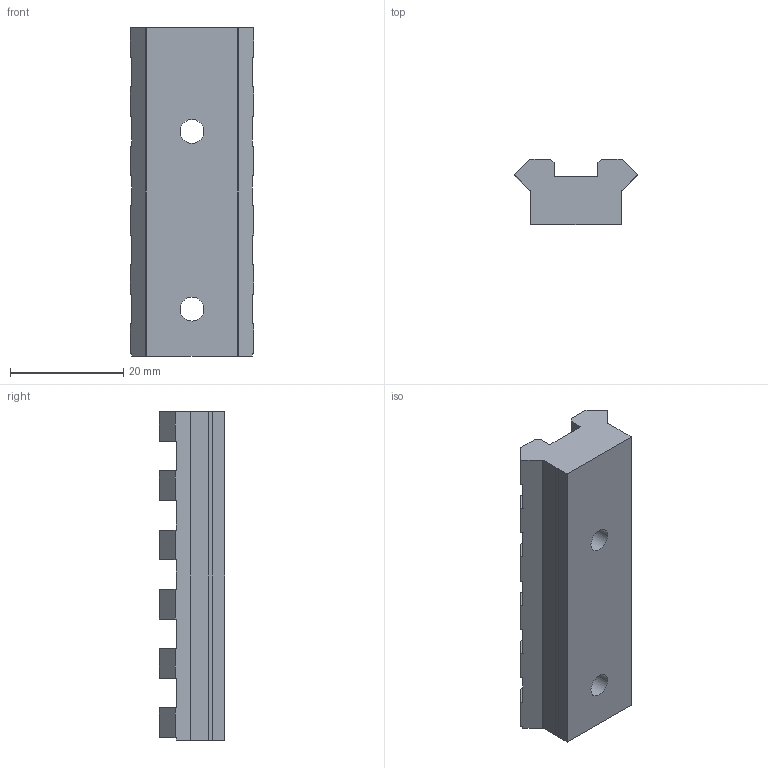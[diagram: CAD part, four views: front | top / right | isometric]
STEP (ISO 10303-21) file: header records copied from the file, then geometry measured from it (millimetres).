
FILE_DESCRIPTION(('FreeCAD Model'),'2;1');
FILE_NAME('ap9 sight rail.step', '2017-07-29T22:49:40',('Author'),(''), 'Open CASCADE STEP processor 6.8','FreeCAD','Unknown');
FILE_SCHEMA(('AUTOMOTIVE_DESIGN_CC2 { 1 2 10303 214 -1 1 5 4 }'));
Length unit declared in the file: millimetre
Products named in the file (1): Pocket003
Bounding box: 21.79 x 11.48 x 57.99 mm (x, y, z)
Volume: 8801.8 mm3; surface area: 4522.7 mm2
Topology: 1 solids, 1 shells, 92 faces, 264 edges, 176 vertices
Faces by surface type: plane 88, cylinder 4
Full cylindrical faces by diameter (mm): 4.2 x2, 8.2 x2
Entity records: 6359 total; most frequent: CARTESIAN_POINT 1173, DIRECTION 904, LINE 700, VECTOR 700, ORIENTED_EDGE 528, PCURVE 528, DEFINITIONAL_REPRESENTATION 528, EDGE_CURVE 264
